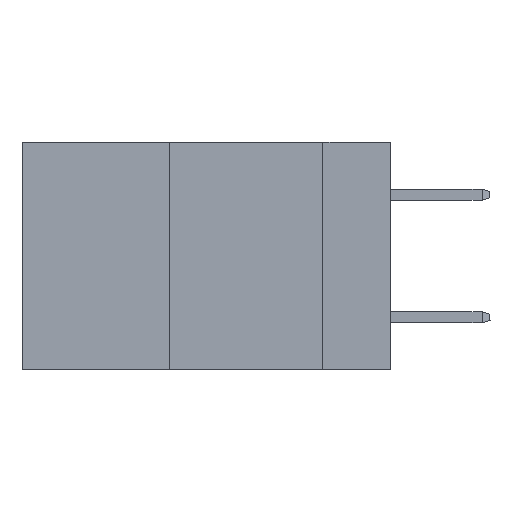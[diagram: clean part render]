
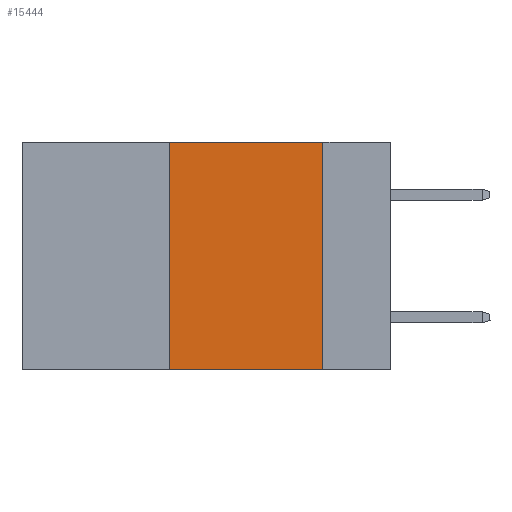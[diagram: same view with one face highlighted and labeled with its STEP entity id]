
A CAD part, left-side view. The second image highlights one B-rep face of the part: STEP entity #15444.
In plain terms, the highlighted planar face has unit normal (-1, 0, 0).
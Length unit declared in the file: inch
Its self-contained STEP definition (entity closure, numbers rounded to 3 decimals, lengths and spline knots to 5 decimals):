
#840 = DIRECTION ( 'NONE',  ( 0., 0., -1. ) ) ;
#846 = CARTESIAN_POINT ( 'NONE',  ( 0., 0.11, -0.37 ) ) ;
#1720 = ORIENTED_EDGE ( 'NONE', *, *, #7291, .F. ) ;
#2177 = LINE ( 'NONE', #9581, #15367 ) ;
#2372 = ORIENTED_EDGE ( 'NONE', *, *, #22673, .T. ) ;
#2516 = DIRECTION ( 'NONE',  ( 0., 0., 1. ) ) ;
#3682 = EDGE_CURVE ( 'NONE', #12876, #19660, #2177, .T. ) ;
#3736 = VECTOR ( 'NONE', #22094, 39.37008 ) ;
#3913 = DIRECTION ( 'NONE',  ( 0., 0., -1. ) ) ;
#4328 = AXIS2_PLACEMENT_3D ( 'NONE', #10804, #21620, #3913 ) ;
#4447 = EDGE_LOOP ( 'NONE', ( #1720, #10679, #15113, #2372 ) ) ;
#5101 = LINE ( 'NONE', #20285, #5367 ) ;
#5367 = VECTOR ( 'NONE', #9551, 39.37008 ) ;
#5558 = LINE ( 'NONE', #11420, #11143 ) ;
#5949 = CARTESIAN_POINT ( 'NONE',  ( 0., 0.6, -0.37 ) ) ;
#7141 = VERTEX_POINT ( 'NONE', #15955 ) ;
#7291 = EDGE_CURVE ( 'NONE', #7141, #21661, #5558, .T. ) ;
#7306 = FACE_OUTER_BOUND ( 'NONE', #4447, .T. ) ;
#9551 = DIRECTION ( 'NONE',  ( 0., -1., 0. ) ) ;
#9581 = CARTESIAN_POINT ( 'NONE',  ( 0., 0.36, 0. ) ) ;
#10679 = ORIENTED_EDGE ( 'NONE', *, *, #10765, .F. ) ;
#10765 = EDGE_CURVE ( 'NONE', #19660, #7141, #5101, .T. ) ;
#10804 = CARTESIAN_POINT ( 'NONE',  ( 0., 0.6, 0. ) ) ;
#10945 = CARTESIAN_POINT ( 'NONE',  ( 0., 0.36, -0.37 ) ) ;
#11143 = VECTOR ( 'NONE', #840, 39.37008 ) ;
#11420 = CARTESIAN_POINT ( 'NONE',  ( 0., 0.11, 0. ) ) ;
#12876 = VERTEX_POINT ( 'NONE', #10945 ) ;
#13179 = CARTESIAN_POINT ( 'NONE',  ( 0., 0.36, 0. ) ) ;
#13495 = LINE ( 'NONE', #5949, #3736 ) ;
#15113 = ORIENTED_EDGE ( 'NONE', *, *, #3682, .F. ) ;
#15367 = VECTOR ( 'NONE', #2516, 39.37008 ) ;
#15444 = ADVANCED_FACE ( 'NONE', ( #7306 ), #16128, .F. ) ;
#15955 = CARTESIAN_POINT ( 'NONE',  ( 0., 0.11, 0. ) ) ;
#16128 = PLANE ( 'NONE',  #4328 ) ;
#19660 = VERTEX_POINT ( 'NONE', #13179 ) ;
#20285 = CARTESIAN_POINT ( 'NONE',  ( 0., 0.6, 0. ) ) ;
#21620 = DIRECTION ( 'NONE',  ( 1., 0., 0. ) ) ;
#21661 = VERTEX_POINT ( 'NONE', #846 ) ;
#22094 = DIRECTION ( 'NONE',  ( 0., -1., 0. ) ) ;
#22673 = EDGE_CURVE ( 'NONE', #12876, #21661, #13495, .T. ) ;
